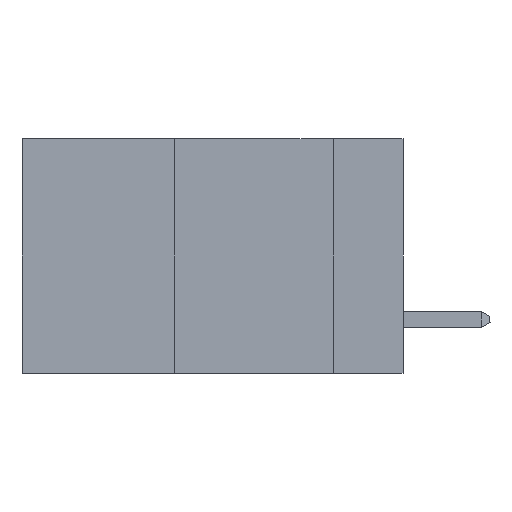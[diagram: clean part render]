
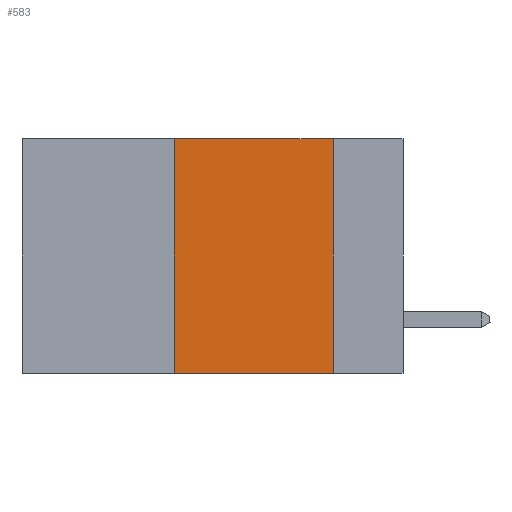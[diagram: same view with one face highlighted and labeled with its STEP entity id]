
A CAD part, left-side view. The second image highlights one B-rep face of the part: STEP entity #583.
In plain terms, the highlighted planar face has unit normal (-1, 0, 0).
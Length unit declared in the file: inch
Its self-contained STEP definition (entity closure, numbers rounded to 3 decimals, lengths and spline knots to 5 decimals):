
#583 = ADVANCED_FACE ( 'NONE', ( #4279 ), #24708, .F. ) ;
#3415 = ORIENTED_EDGE ( 'NONE', *, *, #14496, .T. ) ;
#3774 = VERTEX_POINT ( 'NONE', #10372 ) ;
#4279 = FACE_OUTER_BOUND ( 'NONE', #32207, .T. ) ;
#4359 = DIRECTION ( 'NONE',  ( 1., 0., 0. ) ) ;
#7148 = DIRECTION ( 'NONE',  ( 0., 0., -1. ) ) ;
#8252 = EDGE_CURVE ( 'NONE', #28587, #31815, #36945, .T. ) ;
#8775 = CARTESIAN_POINT ( 'NONE',  ( 0., 0.36, -0.37 ) ) ;
#9932 = CARTESIAN_POINT ( 'NONE',  ( 0., 0.6, -0.37 ) ) ;
#10372 = CARTESIAN_POINT ( 'NONE',  ( 0., 0.11, 0. ) ) ;
#10708 = VECTOR ( 'NONE', #13760, 39.37008 ) ;
#11274 = DIRECTION ( 'NONE',  ( 0., 0., 1. ) ) ;
#12042 = VECTOR ( 'NONE', #15596, 39.37008 ) ;
#13289 = AXIS2_PLACEMENT_3D ( 'NONE', #21911, #4359, #7148 ) ;
#13581 = VECTOR ( 'NONE', #11274, 39.37008 ) ;
#13760 = DIRECTION ( 'NONE',  ( 0., -1., 0. ) ) ;
#14288 = EDGE_CURVE ( 'NONE', #31815, #3774, #29539, .T. ) ;
#14496 = EDGE_CURVE ( 'NONE', #28587, #33238, #17589, .T. ) ;
#15078 = CARTESIAN_POINT ( 'NONE',  ( 0., 0.11, -0.37 ) ) ;
#15596 = DIRECTION ( 'NONE',  ( 0., -1., 0. ) ) ;
#17054 = CARTESIAN_POINT ( 'NONE',  ( 0., 0.6, 0. ) ) ;
#17589 = LINE ( 'NONE', #9932, #12042 ) ;
#18344 = LINE ( 'NONE', #31427, #33999 ) ;
#19323 = CARTESIAN_POINT ( 'NONE',  ( 0., 0.36, 0. ) ) ;
#21911 = CARTESIAN_POINT ( 'NONE',  ( 0., 0.6, 0. ) ) ;
#24708 = PLANE ( 'NONE',  #13289 ) ;
#25311 = ORIENTED_EDGE ( 'NONE', *, *, #14288, .F. ) ;
#25615 = DIRECTION ( 'NONE',  ( 0., 0., -1. ) ) ;
#26263 = ORIENTED_EDGE ( 'NONE', *, *, #32605, .F. ) ;
#28587 = VERTEX_POINT ( 'NONE', #8775 ) ;
#29539 = LINE ( 'NONE', #17054, #10708 ) ;
#30036 = ORIENTED_EDGE ( 'NONE', *, *, #8252, .F. ) ;
#31427 = CARTESIAN_POINT ( 'NONE',  ( 0., 0.11, 0. ) ) ;
#31460 = CARTESIAN_POINT ( 'NONE',  ( 0., 0.36, 0. ) ) ;
#31815 = VERTEX_POINT ( 'NONE', #19323 ) ;
#32207 = EDGE_LOOP ( 'NONE', ( #26263, #25311, #30036, #3415 ) ) ;
#32605 = EDGE_CURVE ( 'NONE', #3774, #33238, #18344, .T. ) ;
#33238 = VERTEX_POINT ( 'NONE', #15078 ) ;
#33999 = VECTOR ( 'NONE', #25615, 39.37008 ) ;
#36945 = LINE ( 'NONE', #31460, #13581 ) ;
